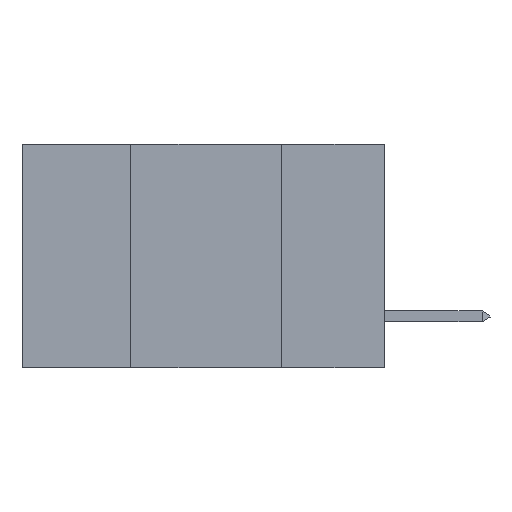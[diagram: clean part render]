
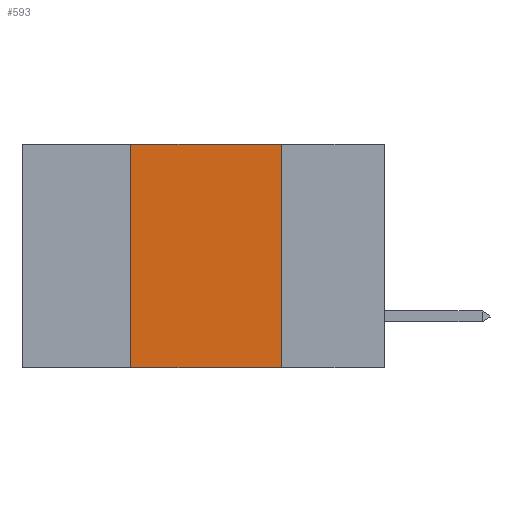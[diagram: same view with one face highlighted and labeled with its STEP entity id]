
A CAD part, left-side view. The second image highlights one B-rep face of the part: STEP entity #593.
In plain terms, the highlighted planar face has unit normal (-1, 0, 0).
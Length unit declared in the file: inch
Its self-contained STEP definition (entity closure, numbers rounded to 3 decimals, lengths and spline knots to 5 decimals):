
#19 = CARTESIAN_POINT ( 'NONE',  ( 0., 0.6, -0.37 ) ) ;
#120 = DIRECTION ( 'NONE',  ( 1., 0., 0. ) ) ;
#176 = PLANE ( 'NONE',  #8955 ) ;
#347 = EDGE_CURVE ( 'NONE', #8726, #12124, #14803, .T. ) ;
#593 = ADVANCED_FACE ( 'NONE', ( #11696 ), #176, .F. ) ;
#792 = VECTOR ( 'NONE', #6368, 39.37008 ) ;
#1235 = EDGE_CURVE ( 'NONE', #8726, #16462, #7267, .T. ) ;
#1489 = CARTESIAN_POINT ( 'NONE',  ( 0., 0.42, -0.37 ) ) ;
#1582 = CARTESIAN_POINT ( 'NONE',  ( 0., 0.6, 0. ) ) ;
#2191 = ORIENTED_EDGE ( 'NONE', *, *, #347, .T. ) ;
#2359 = CARTESIAN_POINT ( 'NONE',  ( 0., 0.17, 0. ) ) ;
#2601 = VECTOR ( 'NONE', #5580, 39.37008 ) ;
#3600 = ORIENTED_EDGE ( 'NONE', *, *, #1235, .F. ) ;
#3794 = LINE ( 'NONE', #12929, #13989 ) ;
#5580 = DIRECTION ( 'NONE',  ( 0., 0., 1. ) ) ;
#5744 = DIRECTION ( 'NONE',  ( 0., 0., -1. ) ) ;
#6368 = DIRECTION ( 'NONE',  ( 0., 0., -1. ) ) ;
#6697 = EDGE_CURVE ( 'NONE', #17740, #12124, #14713, .T. ) ;
#7267 = LINE ( 'NONE', #9170, #2601 ) ;
#7308 = VECTOR ( 'NONE', #10169, 39.37008 ) ;
#8726 = VERTEX_POINT ( 'NONE', #1489 ) ;
#8840 = DIRECTION ( 'NONE',  ( 0., -1., 0. ) ) ;
#8955 = AXIS2_PLACEMENT_3D ( 'NONE', #1582, #120, #5744 ) ;
#9170 = CARTESIAN_POINT ( 'NONE',  ( 0., 0.42, 0. ) ) ;
#10169 = DIRECTION ( 'NONE',  ( 0., -1., 0. ) ) ;
#10314 = ORIENTED_EDGE ( 'NONE', *, *, #6697, .F. ) ;
#11433 = EDGE_LOOP ( 'NONE', ( #10314, #15742, #3600, #2191 ) ) ;
#11696 = FACE_OUTER_BOUND ( 'NONE', #11433, .T. ) ;
#12075 = EDGE_CURVE ( 'NONE', #16462, #17740, #3794, .T. ) ;
#12124 = VERTEX_POINT ( 'NONE', #15654 ) ;
#12929 = CARTESIAN_POINT ( 'NONE',  ( 0., 0.6, 0. ) ) ;
#13989 = VECTOR ( 'NONE', #8840, 39.37008 ) ;
#14713 = LINE ( 'NONE', #16124, #792 ) ;
#14803 = LINE ( 'NONE', #19, #7308 ) ;
#14995 = CARTESIAN_POINT ( 'NONE',  ( 0., 0.42, 0. ) ) ;
#15654 = CARTESIAN_POINT ( 'NONE',  ( 0., 0.17, -0.37 ) ) ;
#15742 = ORIENTED_EDGE ( 'NONE', *, *, #12075, .F. ) ;
#16124 = CARTESIAN_POINT ( 'NONE',  ( 0., 0.17, 0. ) ) ;
#16462 = VERTEX_POINT ( 'NONE', #14995 ) ;
#17740 = VERTEX_POINT ( 'NONE', #2359 ) ;
